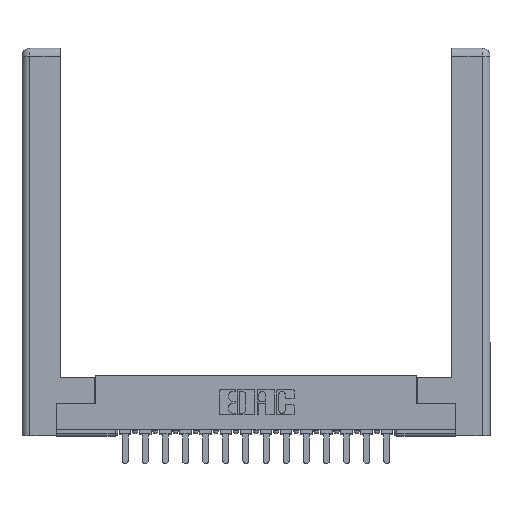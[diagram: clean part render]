
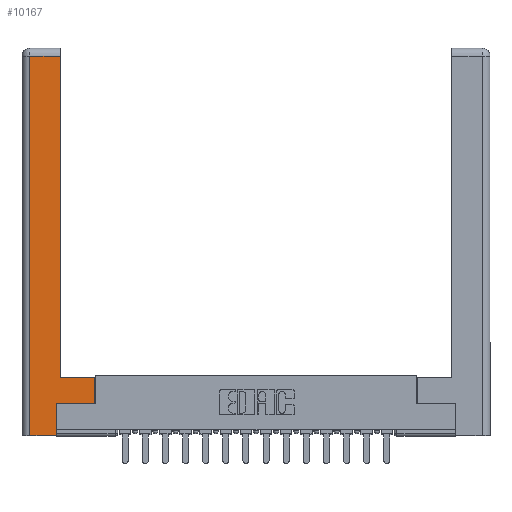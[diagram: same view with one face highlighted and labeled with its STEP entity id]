
A CAD part, top view. The second image highlights one B-rep face of the part: STEP entity #10167.
In plain terms, the highlighted planar face has unit normal (0, 0, 1).
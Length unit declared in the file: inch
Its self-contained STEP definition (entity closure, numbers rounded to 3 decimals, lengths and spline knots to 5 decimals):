
#230 = CARTESIAN_POINT ( 'NONE',  ( 0.0615, 0., 0. ) ) ;
#617 = CARTESIAN_POINT ( 'NONE',  ( 0.0615, 2.94, 0. ) ) ;
#1161 = CARTESIAN_POINT ( 'NONE',  ( 0.0615, 0., 0. ) ) ;
#1196 = EDGE_CURVE ( 'NONE', #8743, #15681, #2008, .T. ) ;
#1363 = LINE ( 'NONE', #1161, #16064 ) ;
#1711 = FACE_OUTER_BOUND ( 'NONE', #15534, .T. ) ;
#1983 = VERTEX_POINT ( 'NONE', #6362 ) ;
#2008 = LINE ( 'NONE', #4975, #10549 ) ;
#2334 = ORIENTED_EDGE ( 'NONE', *, *, #3908, .T. ) ;
#2407 = LINE ( 'NONE', #12625, #10071 ) ;
#2483 = CARTESIAN_POINT ( 'NONE',  ( 0.295, 0.45, 0. ) ) ;
#2756 = EDGE_CURVE ( 'NONE', #15618, #17963, #1363, .T. ) ;
#2932 = ORIENTED_EDGE ( 'NONE', *, *, #10716, .T. ) ;
#3001 = ORIENTED_EDGE ( 'NONE', *, *, #2756, .T. ) ;
#3469 = EDGE_CURVE ( 'NONE', #1983, #8743, #7034, .T. ) ;
#3482 = LINE ( 'NONE', #12271, #9526 ) ;
#3879 = CARTESIAN_POINT ( 'NONE',  ( 0.565, 0.245, 0. ) ) ;
#3908 = EDGE_CURVE ( 'NONE', #17963, #16002, #8434, .T. ) ;
#4975 = CARTESIAN_POINT ( 'NONE',  ( 0.295, 3., 0. ) ) ;
#5548 = VERTEX_POINT ( 'NONE', #16629 ) ;
#5690 = CARTESIAN_POINT ( 'NONE',  ( 0.295, 0.45, 0. ) ) ;
#6098 = DIRECTION ( 'NONE',  ( -1., 0., 0. ) ) ;
#6239 = CARTESIAN_POINT ( 'NONE',  ( 0.295, 2.94, 0. ) ) ;
#6362 = CARTESIAN_POINT ( 'NONE',  ( 0.565, 0.45, 0. ) ) ;
#6870 = DIRECTION ( 'NONE',  ( 0., 1., 0. ) ) ;
#6961 = VECTOR ( 'NONE', #17123, 39.37008 ) ;
#7034 = LINE ( 'NONE', #5690, #6961 ) ;
#7278 = CARTESIAN_POINT ( 'NONE',  ( 0.265, 0., 0. ) ) ;
#7535 = PLANE ( 'NONE',  #17687 ) ;
#8173 = VECTOR ( 'NONE', #15779, 39.37008 ) ;
#8434 = LINE ( 'NONE', #10164, #8173 ) ;
#8672 = LINE ( 'NONE', #18816, #12289 ) ;
#8743 = VERTEX_POINT ( 'NONE', #2483 ) ;
#9311 = DIRECTION ( 'NONE',  ( -1., 0., 0. ) ) ;
#9526 = VECTOR ( 'NONE', #18231, 39.37008 ) ;
#9871 = DIRECTION ( 'NONE',  ( 1., 0., 0. ) ) ;
#10071 = VECTOR ( 'NONE', #9871, 39.37008 ) ;
#10164 = CARTESIAN_POINT ( 'NONE',  ( 0.265, 0., 0. ) ) ;
#10167 = ADVANCED_FACE ( 'NONE', ( #1711 ), #7535, .F. ) ;
#10222 = DIRECTION ( 'NONE',  ( 0., 0., -1. ) ) ;
#10253 = ORIENTED_EDGE ( 'NONE', *, *, #1196, .T. ) ;
#10549 = VECTOR ( 'NONE', #10809, 39.37008 ) ;
#10716 = EDGE_CURVE ( 'NONE', #15458, #1983, #3482, .T. ) ;
#10809 = DIRECTION ( 'NONE',  ( 0., 1., 0. ) ) ;
#11088 = VECTOR ( 'NONE', #9311, 39.37008 ) ;
#11269 = ORIENTED_EDGE ( 'NONE', *, *, #15733, .T. ) ;
#11381 = ORIENTED_EDGE ( 'NONE', *, *, #3469, .T. ) ;
#11501 = ORIENTED_EDGE ( 'NONE', *, *, #11987, .T. ) ;
#11634 = ORIENTED_EDGE ( 'NONE', *, *, #11681, .T. ) ;
#11681 = EDGE_CURVE ( 'NONE', #16002, #5548, #8672, .T. ) ;
#11987 = EDGE_CURVE ( 'NONE', #15681, #15618, #12173, .T. ) ;
#12173 = LINE ( 'NONE', #617, #11088 ) ;
#12271 = CARTESIAN_POINT ( 'NONE',  ( 0.565, 0.45, 0. ) ) ;
#12289 = VECTOR ( 'NONE', #6870, 39.37008 ) ;
#12338 = CARTESIAN_POINT ( 'NONE',  ( 0.0615, 2.94, 0. ) ) ;
#12625 = CARTESIAN_POINT ( 'NONE',  ( 0.565, 0.245, 0. ) ) ;
#13349 = CARTESIAN_POINT ( 'NONE',  ( 0., 0., 0. ) ) ;
#15458 = VERTEX_POINT ( 'NONE', #3879 ) ;
#15534 = EDGE_LOOP ( 'NONE', ( #10253, #11501, #3001, #2334, #11634, #11269, #2932, #11381 ) ) ;
#15618 = VERTEX_POINT ( 'NONE', #12338 ) ;
#15681 = VERTEX_POINT ( 'NONE', #6239 ) ;
#15733 = EDGE_CURVE ( 'NONE', #5548, #15458, #2407, .T. ) ;
#15779 = DIRECTION ( 'NONE',  ( 1., 0., 0. ) ) ;
#16002 = VERTEX_POINT ( 'NONE', #7278 ) ;
#16064 = VECTOR ( 'NONE', #18775, 39.37008 ) ;
#16629 = CARTESIAN_POINT ( 'NONE',  ( 0.265, 0.245, 0. ) ) ;
#17123 = DIRECTION ( 'NONE',  ( -1., 0., 0. ) ) ;
#17687 = AXIS2_PLACEMENT_3D ( 'NONE', #13349, #10222, #6098 ) ;
#17963 = VERTEX_POINT ( 'NONE', #230 ) ;
#18231 = DIRECTION ( 'NONE',  ( 0., 1., 0. ) ) ;
#18775 = DIRECTION ( 'NONE',  ( 0., -1., 0. ) ) ;
#18816 = CARTESIAN_POINT ( 'NONE',  ( 0.265, 0.245, 0. ) ) ;
